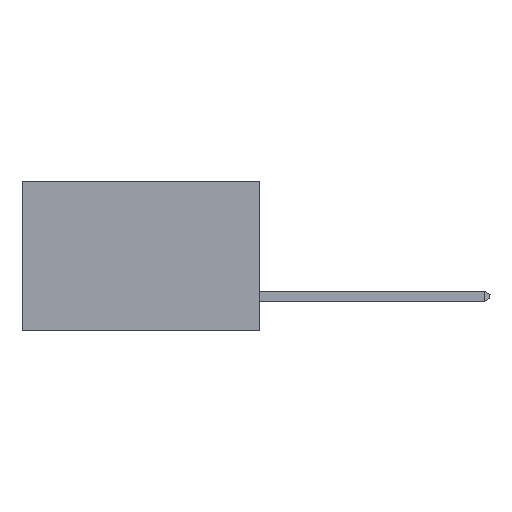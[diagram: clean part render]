
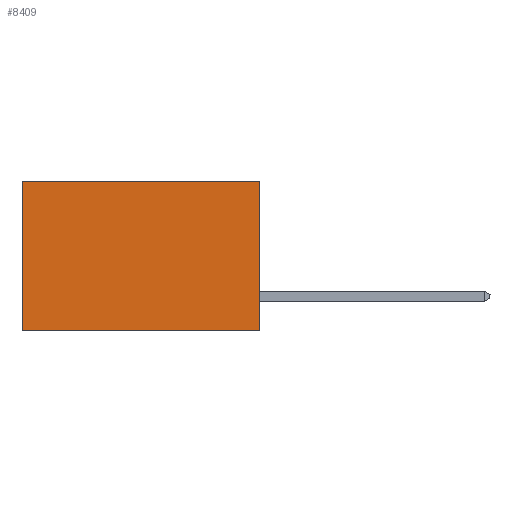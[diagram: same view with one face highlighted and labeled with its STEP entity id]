
A CAD part, left-side view. The second image highlights one B-rep face of the part: STEP entity #8409.
In plain terms, the highlighted planar face has unit normal (-1, 0, 0).
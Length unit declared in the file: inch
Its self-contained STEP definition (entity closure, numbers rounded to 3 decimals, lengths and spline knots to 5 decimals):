
#25 = LINE ( 'NONE', #1035, #3428 ) ;
#340 = CARTESIAN_POINT ( 'NONE',  ( 0.277, 0., -0.37 ) ) ;
#415 = CARTESIAN_POINT ( 'NONE',  ( 0.277, 0., 0. ) ) ;
#577 = CARTESIAN_POINT ( 'NONE',  ( 0.277, 0.59, 0. ) ) ;
#632 = CARTESIAN_POINT ( 'NONE',  ( 0.277, 0., -0.37 ) ) ;
#765 = ORIENTED_EDGE ( 'NONE', *, *, #1538, .F. ) ;
#1014 = DIRECTION ( 'NONE',  ( 0., 0., -1. ) ) ;
#1035 = CARTESIAN_POINT ( 'NONE',  ( 0.277, 0., -0.37 ) ) ;
#1084 = DIRECTION ( 'NONE',  ( 0., 1., 0. ) ) ;
#1148 = CARTESIAN_POINT ( 'NONE',  ( 0.277, 0.59, -0.37 ) ) ;
#1296 = DIRECTION ( 'NONE',  ( 0., 0., -1. ) ) ;
#1301 = CARTESIAN_POINT ( 'NONE',  ( 0.277, 0., 0. ) ) ;
#1488 = VERTEX_POINT ( 'NONE', #1148 ) ;
#1538 = EDGE_CURVE ( 'NONE', #2825, #8708, #25, .T. ) ;
#1903 = LINE ( 'NONE', #2974, #3734 ) ;
#2150 = ORIENTED_EDGE ( 'NONE', *, *, #6999, .F. ) ;
#2825 = VERTEX_POINT ( 'NONE', #1301 ) ;
#2974 = CARTESIAN_POINT ( 'NONE',  ( 0.277, 0.59, -0.37 ) ) ;
#3428 = VECTOR ( 'NONE', #1296, 39.37008 ) ;
#3562 = EDGE_LOOP ( 'NONE', ( #6913, #2150, #765, #6812 ) ) ;
#3733 = PLANE ( 'NONE',  #7773 ) ;
#3734 = VECTOR ( 'NONE', #7662, 39.37008 ) ;
#4061 = CARTESIAN_POINT ( 'NONE',  ( 0.277, 0., -0.37 ) ) ;
#5122 = DIRECTION ( 'NONE',  ( 1., 0., 0. ) ) ;
#5233 = FACE_OUTER_BOUND ( 'NONE', #3562, .T. ) ;
#5355 = VECTOR ( 'NONE', #1084, 39.37008 ) ;
#5940 = VERTEX_POINT ( 'NONE', #577 ) ;
#6735 = DIRECTION ( 'NONE',  ( 0., 1., 0. ) ) ;
#6812 = ORIENTED_EDGE ( 'NONE', *, *, #7372, .T. ) ;
#6910 = VECTOR ( 'NONE', #6735, 39.37008 ) ;
#6913 = ORIENTED_EDGE ( 'NONE', *, *, #7727, .T. ) ;
#6999 = EDGE_CURVE ( 'NONE', #8708, #1488, #8441, .T. ) ;
#7111 = LINE ( 'NONE', #415, #5355 ) ;
#7372 = EDGE_CURVE ( 'NONE', #2825, #5940, #7111, .T. ) ;
#7662 = DIRECTION ( 'NONE',  ( 0., 0., -1. ) ) ;
#7727 = EDGE_CURVE ( 'NONE', #5940, #1488, #1903, .T. ) ;
#7773 = AXIS2_PLACEMENT_3D ( 'NONE', #340, #5122, #1014 ) ;
#8409 = ADVANCED_FACE ( 'NONE', ( #5233 ), #3733, .F. ) ;
#8441 = LINE ( 'NONE', #632, #6910 ) ;
#8708 = VERTEX_POINT ( 'NONE', #4061 ) ;
